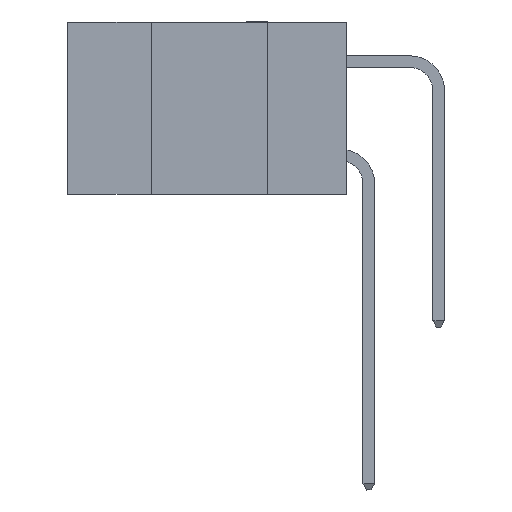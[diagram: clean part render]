
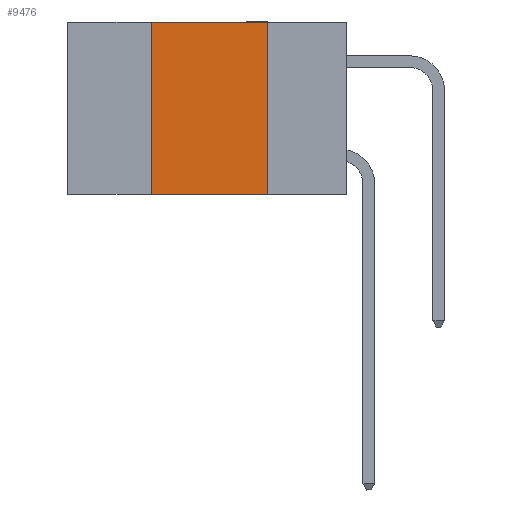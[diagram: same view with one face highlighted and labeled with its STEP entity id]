
A CAD part, left-side view. The second image highlights one B-rep face of the part: STEP entity #9476.
In plain terms, the highlighted planar face has unit normal (-1, 0, 0).
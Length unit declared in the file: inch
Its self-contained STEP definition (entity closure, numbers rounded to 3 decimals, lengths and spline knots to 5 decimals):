
#299 = ORIENTED_EDGE ( 'NONE', *, *, #12813, .F. ) ;
#2163 = VERTEX_POINT ( 'NONE', #11122 ) ;
#3381 = CARTESIAN_POINT ( 'NONE',  ( 0., 0.6, -0.37 ) ) ;
#3579 = DIRECTION ( 'NONE',  ( 0., -1., 0. ) ) ;
#4169 = VECTOR ( 'NONE', #6317, 39.37008 ) ;
#4622 = VERTEX_POINT ( 'NONE', #6759 ) ;
#5035 = ORIENTED_EDGE ( 'NONE', *, *, #7425, .T. ) ;
#5099 = DIRECTION ( 'NONE',  ( 0., 0., 1. ) ) ;
#5200 = VERTEX_POINT ( 'NONE', #5371 ) ;
#5371 = CARTESIAN_POINT ( 'NONE',  ( 0., 0.17, -0.37 ) ) ;
#5774 = PLANE ( 'NONE',  #11729 ) ;
#5779 = LINE ( 'NONE', #10731, #4169 ) ;
#5940 = VECTOR ( 'NONE', #3579, 39.37008 ) ;
#6317 = DIRECTION ( 'NONE',  ( 0., -1., 0. ) ) ;
#6670 = EDGE_CURVE ( 'NONE', #4622, #16771, #11036, .T. ) ;
#6759 = CARTESIAN_POINT ( 'NONE',  ( 0., 0.42, -0.37 ) ) ;
#7160 = ORIENTED_EDGE ( 'NONE', *, *, #6670, .F. ) ;
#7425 = EDGE_CURVE ( 'NONE', #4622, #5200, #9869, .T. ) ;
#8200 = DIRECTION ( 'NONE',  ( 0., 0., -1. ) ) ;
#9417 = CARTESIAN_POINT ( 'NONE',  ( 0., 0.42, 0. ) ) ;
#9476 = ADVANCED_FACE ( 'NONE', ( #18253 ), #5774, .F. ) ;
#9772 = CARTESIAN_POINT ( 'NONE',  ( 0., 0.42, 0. ) ) ;
#9869 = LINE ( 'NONE', #3381, #5940 ) ;
#10058 = ORIENTED_EDGE ( 'NONE', *, *, #12286, .F. ) ;
#10183 = VECTOR ( 'NONE', #8200, 39.37008 ) ;
#10731 = CARTESIAN_POINT ( 'NONE',  ( 0., 0.6, 0. ) ) ;
#11036 = LINE ( 'NONE', #9417, #18375 ) ;
#11122 = CARTESIAN_POINT ( 'NONE',  ( 0., 0.17, 0. ) ) ;
#11729 = AXIS2_PLACEMENT_3D ( 'NONE', #14510, #14632, #17585 ) ;
#12286 = EDGE_CURVE ( 'NONE', #2163, #5200, #12703, .T. ) ;
#12482 = EDGE_LOOP ( 'NONE', ( #10058, #299, #7160, #5035 ) ) ;
#12703 = LINE ( 'NONE', #18339, #10183 ) ;
#12813 = EDGE_CURVE ( 'NONE', #16771, #2163, #5779, .T. ) ;
#14510 = CARTESIAN_POINT ( 'NONE',  ( 0., 0.6, 0. ) ) ;
#14632 = DIRECTION ( 'NONE',  ( 1., 0., 0. ) ) ;
#16771 = VERTEX_POINT ( 'NONE', #9772 ) ;
#17585 = DIRECTION ( 'NONE',  ( 0., 0., -1. ) ) ;
#18253 = FACE_OUTER_BOUND ( 'NONE', #12482, .T. ) ;
#18339 = CARTESIAN_POINT ( 'NONE',  ( 0., 0.17, 0. ) ) ;
#18375 = VECTOR ( 'NONE', #5099, 39.37008 ) ;
